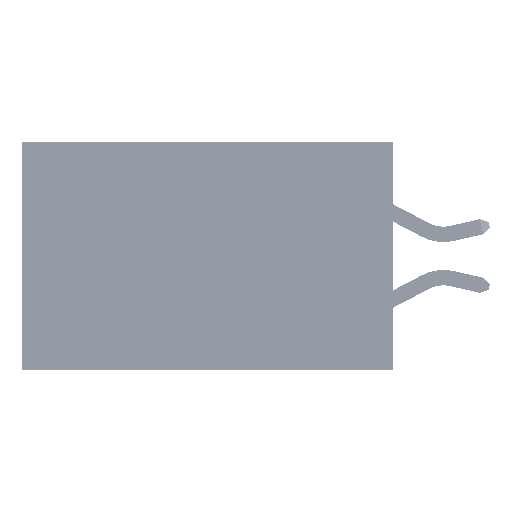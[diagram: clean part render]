
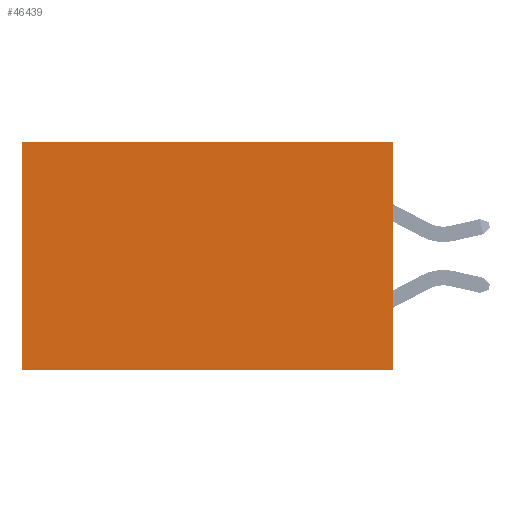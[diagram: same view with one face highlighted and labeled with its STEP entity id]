
A CAD part, left-side view. The second image highlights one B-rep face of the part: STEP entity #46439.
In plain terms, the highlighted planar face has unit normal (-1, 0, 0).
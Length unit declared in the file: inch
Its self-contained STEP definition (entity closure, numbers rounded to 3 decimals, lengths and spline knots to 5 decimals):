
#529 = ORIENTED_EDGE ( 'NONE', *, *, #32206, .F. ) ;
#695 = PLANE ( 'NONE',  #9233 ) ;
#3966 = FACE_OUTER_BOUND ( 'NONE', #29697, .T. ) ;
#6834 = VECTOR ( 'NONE', #23572, 39.37008 ) ;
#7126 = VERTEX_POINT ( 'NONE', #17844 ) ;
#7543 = ORIENTED_EDGE ( 'NONE', *, *, #30810, .T. ) ;
#7977 = VERTEX_POINT ( 'NONE', #35843 ) ;
#9233 = AXIS2_PLACEMENT_3D ( 'NONE', #22829, #19183, #26898 ) ;
#9600 = CARTESIAN_POINT ( 'NONE',  ( 0.2875, 0.6, 0. ) ) ;
#10760 = VECTOR ( 'NONE', #13515, 39.37008 ) ;
#13515 = DIRECTION ( 'NONE',  ( 0., 0., -1. ) ) ;
#16159 = VECTOR ( 'NONE', #48026, 39.37008 ) ;
#16321 = EDGE_CURVE ( 'NONE', #7126, #35823, #17414, .T. ) ;
#17414 = LINE ( 'NONE', #38820, #6834 ) ;
#17844 = CARTESIAN_POINT ( 'NONE',  ( 0.2875, 0., 0. ) ) ;
#19183 = DIRECTION ( 'NONE',  ( 1., 0., 0. ) ) ;
#21983 = CARTESIAN_POINT ( 'NONE',  ( 0.2875, 0., -0.37 ) ) ;
#22829 = CARTESIAN_POINT ( 'NONE',  ( 0.2875, 0., 0. ) ) ;
#22933 = EDGE_CURVE ( 'NONE', #7977, #29886, #34341, .T. ) ;
#23464 = ORIENTED_EDGE ( 'NONE', *, *, #16321, .T. ) ;
#23572 = DIRECTION ( 'NONE',  ( 0., 1., 0. ) ) ;
#24107 = VECTOR ( 'NONE', #25211, 39.37008 ) ;
#25211 = DIRECTION ( 'NONE',  ( 0., 0., -1. ) ) ;
#26898 = DIRECTION ( 'NONE',  ( 0., 0., -1. ) ) ;
#29697 = EDGE_LOOP ( 'NONE', ( #7543, #46875, #529, #23464 ) ) ;
#29886 = VERTEX_POINT ( 'NONE', #48264 ) ;
#30810 = EDGE_CURVE ( 'NONE', #35823, #29886, #40690, .T. ) ;
#32206 = EDGE_CURVE ( 'NONE', #7126, #7977, #38187, .T. ) ;
#34341 = LINE ( 'NONE', #21983, #16159 ) ;
#35823 = VERTEX_POINT ( 'NONE', #48120 ) ;
#35843 = CARTESIAN_POINT ( 'NONE',  ( 0.2875, 0., -0.37 ) ) ;
#38187 = LINE ( 'NONE', #47818, #24107 ) ;
#38820 = CARTESIAN_POINT ( 'NONE',  ( 0.2875, 0., 0. ) ) ;
#40690 = LINE ( 'NONE', #9600, #10760 ) ;
#46439 = ADVANCED_FACE ( 'NONE', ( #3966 ), #695, .F. ) ;
#46875 = ORIENTED_EDGE ( 'NONE', *, *, #22933, .F. ) ;
#47818 = CARTESIAN_POINT ( 'NONE',  ( 0.2875, 0., 0. ) ) ;
#48026 = DIRECTION ( 'NONE',  ( 0., 1., 0. ) ) ;
#48120 = CARTESIAN_POINT ( 'NONE',  ( 0.2875, 0.6, 0. ) ) ;
#48264 = CARTESIAN_POINT ( 'NONE',  ( 0.2875, 0.6, -0.37 ) ) ;
